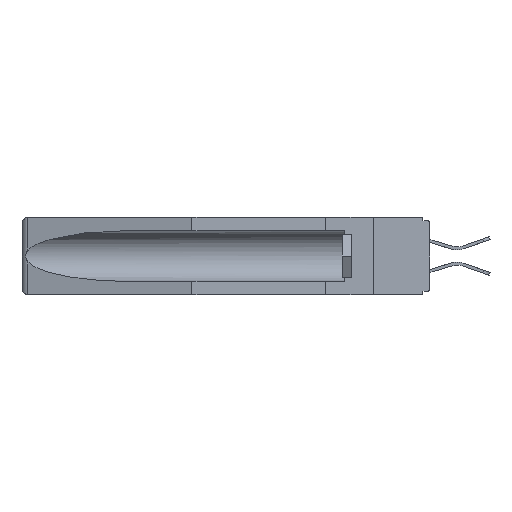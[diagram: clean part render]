
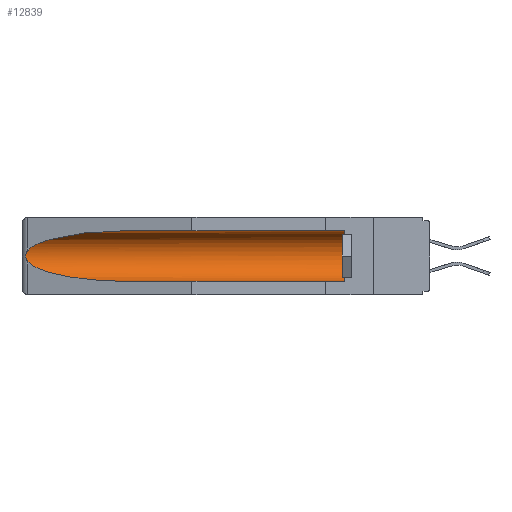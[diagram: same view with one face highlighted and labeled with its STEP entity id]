
A CAD part, left-side view. The second image highlights one B-rep face of the part: STEP entity #12839.
In plain terms, the highlighted cylindrical face has radius 2.857 mm (diameter 5.715 mm), a partial arc.
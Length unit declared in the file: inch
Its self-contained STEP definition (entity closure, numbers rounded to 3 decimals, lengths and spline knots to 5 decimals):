
#188 = EDGE_CURVE ( 'NONE', #11186, #7060, #2017, .T. ) ;
#535 = CIRCLE ( 'NONE', #15146, 0.1125 ) ;
#1504 =( BOUNDED_CURVE ( )  B_SPLINE_CURVE ( 3, ( #25579, #25748, #17010, #13012 ),
 .UNSPECIFIED., .F., .F. ) 
 B_SPLINE_CURVE_WITH_KNOTS ( ( 4, 4 ),
 ( 0.1948, 1.5708 ),
 .UNSPECIFIED. ) 
 CURVE ( )  GEOMETRIC_REPRESENTATION_ITEM ( )  RATIONAL_B_SPLINE_CURVE ( ( 1., 0.848, 0.848, 1. ) ) 
 REPRESENTATION_ITEM ( '' )  );
#1598 = VECTOR ( 'NONE', #26541, 39.37008 ) ;
#1759 = CARTESIAN_POINT ( 'NONE',  ( 0.26537, 1.52718, -0.19328 ) ) ;
#2017 = LINE ( 'NONE', #27186, #26155 ) ;
#2866 = CARTESIAN_POINT ( 'NONE',  ( 0.25451, 1.48313, -0.09465 ) ) ;
#3860 = CARTESIAN_POINT ( 'NONE',  ( 0.2675, 1.53308, -0.17534 ) ) ;
#4428 = EDGE_CURVE ( 'NONE', #10517, #17902, #1504, .T. ) ;
#5728 = FACE_OUTER_BOUND ( 'NONE', #22088, .T. ) ;
#5941 = DIRECTION ( 'NONE',  ( 0., 1., 0. ) ) ;
#6162 = CARTESIAN_POINT ( 'NONE',  ( 0.155, 0.126, -0.284 ) ) ;
#6179 = CARTESIAN_POINT ( 'NONE',  ( 0.155, 0.126, -0.1715 ) ) ;
#6202 = CARTESIAN_POINT ( 'NONE',  ( 0.26537, 1.52718, -0.14972 ) ) ;
#6291 = CARTESIAN_POINT ( 'NONE',  ( 0.2673, 1.5327, -0.16383 ) ) ;
#7060 = VERTEX_POINT ( 'NONE', #16501 ) ;
#7238 = LINE ( 'NONE', #20161, #1598 ) ;
#7318 = CARTESIAN_POINT ( 'NONE',  ( 0.21114, 1.30732, -0.059 ) ) ;
#7436 = B_SPLINE_CURVE_WITH_KNOTS ( 'NONE', 3,
 ( #6202, #12496, #14429, #6291, #8509, #3860, #18680, #8137, #16839, #1759 ),
 .UNSPECIFIED., .F., .F.,
 ( 4, 2, 2, 2, 4 ),
 ( 0., 0.00029, 0.00058, 0.00087, 0.00117 ),
 .UNSPECIFIED. ) ;
#8137 = CARTESIAN_POINT ( 'NONE',  ( 0.26655, 1.53094, -0.18657 ) ) ;
#8221 = VERTEX_POINT ( 'NONE', #6162 ) ;
#8456 = EDGE_CURVE ( 'NONE', #8221, #17902, #7238, .T. ) ;
#8509 = CARTESIAN_POINT ( 'NONE',  ( 0.2675, 1.53308, -0.16763 ) ) ;
#8551 = CARTESIAN_POINT ( 'NONE',  ( 0.155, 1.07973, -0.284 ) ) ;
#9377 = AXIS2_PLACEMENT_3D ( 'NONE', #16309, #5941, #12337 ) ;
#10293 = ORIENTED_EDGE ( 'NONE', *, *, #8456, .F. ) ;
#10517 = VERTEX_POINT ( 'NONE', #14602 ) ;
#10624 = ORIENTED_EDGE ( 'NONE', *, *, #24511, .T. ) ;
#11186 = VERTEX_POINT ( 'NONE', #14153 ) ;
#12201 = DIRECTION ( 'NONE',  ( 0., -1., 0. ) ) ;
#12337 = DIRECTION ( 'NONE',  ( 0., 0., 1. ) ) ;
#12496 = CARTESIAN_POINT ( 'NONE',  ( 0.26597, 1.52961, -0.15275 ) ) ;
#12839 = ADVANCED_FACE ( 'NONE', ( #5728 ), #18612, .F. ) ;
#13012 = CARTESIAN_POINT ( 'NONE',  ( 0.155, 1.07973, -0.284 ) ) ;
#13413 = CARTESIAN_POINT ( 'NONE',  ( 0.26537, 1.52718, -0.14972 ) ) ;
#14153 = CARTESIAN_POINT ( 'NONE',  ( 0.155, 0.126, -0.059 ) ) ;
#14319 = DIRECTION ( 'NONE',  ( 0., 0., 1. ) ) ;
#14429 = CARTESIAN_POINT ( 'NONE',  ( 0.26654, 1.53092, -0.15636 ) ) ;
#14602 = CARTESIAN_POINT ( 'NONE',  ( 0.26537, 1.52718, -0.19328 ) ) ;
#15146 = AXIS2_PLACEMENT_3D ( 'NONE', #6179, #12201, #14319 ) ;
#16309 = CARTESIAN_POINT ( 'NONE',  ( 0.155, -0.30754, -0.1715 ) ) ;
#16501 = CARTESIAN_POINT ( 'NONE',  ( 0.155, 1.07973, -0.059 ) ) ;
#16803 = VERTEX_POINT ( 'NONE', #20801 ) ;
#16839 = CARTESIAN_POINT ( 'NONE',  ( 0.26597, 1.5296, -0.19026 ) ) ;
#17010 = CARTESIAN_POINT ( 'NONE',  ( 0.21114, 1.30732, -0.284 ) ) ;
#17902 = VERTEX_POINT ( 'NONE', #8551 ) ;
#18183 = EDGE_CURVE ( 'NONE', #7060, #16803, #25044, .T. ) ;
#18612 = CYLINDRICAL_SURFACE ( 'NONE', #9377, 0.1125 ) ;
#18680 = CARTESIAN_POINT ( 'NONE',  ( 0.2673, 1.53269, -0.17917 ) ) ;
#19832 = EDGE_CURVE ( 'NONE', #8221, #11186, #535, .T. ) ;
#19970 = ORIENTED_EDGE ( 'NONE', *, *, #18183, .T. ) ;
#20161 = CARTESIAN_POINT ( 'NONE',  ( 0.155, -0.30754, -0.284 ) ) ;
#20801 = CARTESIAN_POINT ( 'NONE',  ( 0.26537, 1.52718, -0.14972 ) ) ;
#22088 = EDGE_LOOP ( 'NONE', ( #19970, #10624, #22896, #10293, #25901, #23277 ) ) ;
#22896 = ORIENTED_EDGE ( 'NONE', *, *, #4428, .T. ) ;
#23277 = ORIENTED_EDGE ( 'NONE', *, *, #188, .T. ) ;
#24511 = EDGE_CURVE ( 'NONE', #16803, #10517, #7436, .T. ) ;
#25044 =( BOUNDED_CURVE ( )  B_SPLINE_CURVE ( 3, ( #26081, #7318, #2866, #13413 ),
 .UNSPECIFIED., .F., .F. ) 
 B_SPLINE_CURVE_WITH_KNOTS ( ( 4, 4 ),
 ( 4.71239, 6.08839 ),
 .UNSPECIFIED. ) 
 CURVE ( )  GEOMETRIC_REPRESENTATION_ITEM ( )  RATIONAL_B_SPLINE_CURVE ( ( 1., 0.848, 0.848, 1. ) ) 
 REPRESENTATION_ITEM ( '' )  );
#25579 = CARTESIAN_POINT ( 'NONE',  ( 0.26537, 1.52718, -0.19328 ) ) ;
#25748 = CARTESIAN_POINT ( 'NONE',  ( 0.25451, 1.48313, -0.24835 ) ) ;
#25901 = ORIENTED_EDGE ( 'NONE', *, *, #19832, .T. ) ;
#26081 = CARTESIAN_POINT ( 'NONE',  ( 0.155, 1.07973, -0.059 ) ) ;
#26155 = VECTOR ( 'NONE', #27375, 39.37008 ) ;
#26541 = DIRECTION ( 'NONE',  ( 0., 1., 0. ) ) ;
#27186 = CARTESIAN_POINT ( 'NONE',  ( 0.155, -0.30754, -0.059 ) ) ;
#27375 = DIRECTION ( 'NONE',  ( 0., 1., 0. ) ) ;
